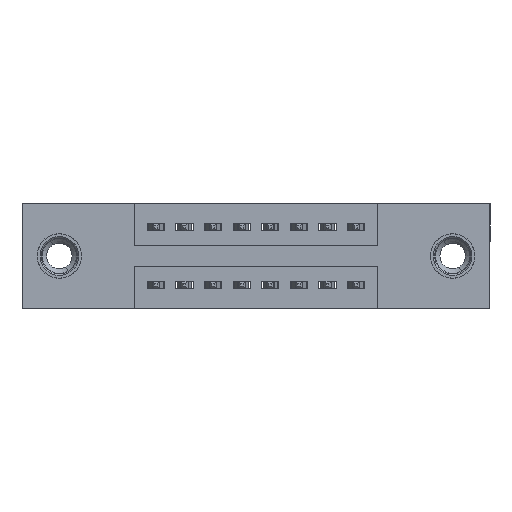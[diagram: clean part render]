
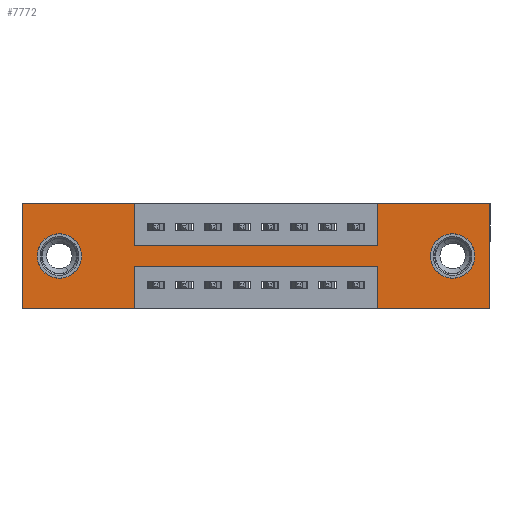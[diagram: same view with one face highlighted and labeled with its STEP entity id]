
A CAD part, front view. The second image highlights one B-rep face of the part: STEP entity #7772.
In plain terms, the highlighted planar face has unit normal (0, -1, 0).
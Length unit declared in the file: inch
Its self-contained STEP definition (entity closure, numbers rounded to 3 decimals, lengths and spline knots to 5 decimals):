
#98 = CARTESIAN_POINT ( 'NONE',  ( 1.505, 0., -0.263 ) ) ;
#171 = VERTEX_POINT ( 'NONE', #9430 ) ;
#197 = CARTESIAN_POINT ( 'NONE',  ( 0.3925, 0., -0.22 ) ) ;
#259 = CARTESIAN_POINT ( 'NONE',  ( 0.3925, 0., 0. ) ) ;
#315 = ORIENTED_EDGE ( 'NONE', *, *, #6123, .F. ) ;
#361 = ORIENTED_EDGE ( 'NONE', *, *, #10981, .F. ) ;
#428 = PLANE ( 'NONE',  #2234 ) ;
#463 = VERTEX_POINT ( 'NONE', #259 ) ;
#629 = ORIENTED_EDGE ( 'NONE', *, *, #6668, .F. ) ;
#678 = VERTEX_POINT ( 'NONE', #6455 ) ;
#683 = VERTEX_POINT ( 'NONE', #7192 ) ;
#689 = EDGE_CURVE ( 'NONE', #10946, #683, #7999, .T. ) ;
#776 = CARTESIAN_POINT ( 'NONE',  ( 1.635, 0., 0. ) ) ;
#910 = CARTESIAN_POINT ( 'NONE',  ( 0., 0., -0.37 ) ) ;
#1120 = VECTOR ( 'NONE', #7804, 39.37008 ) ;
#1314 = EDGE_LOOP ( 'NONE', ( #10425, #361, #12833, #1777, #12569, #7630, #11711, #629, #7399, #3839, #2963, #315 ) ) ;
#1713 = DIRECTION ( 'NONE',  ( 1., 0., 0. ) ) ;
#1764 = CARTESIAN_POINT ( 'NONE',  ( 1.505, 0., -0.185 ) ) ;
#1777 = ORIENTED_EDGE ( 'NONE', *, *, #10527, .F. ) ;
#1779 = DIRECTION ( 'NONE',  ( 1., 0., 0. ) ) ;
#1826 = EDGE_CURVE ( 'NONE', #463, #171, #8135, .T. ) ;
#1947 = EDGE_CURVE ( 'NONE', #9766, #4601, #3247, .T. ) ;
#1992 = DIRECTION ( 'NONE',  ( 0., 0., -1. ) ) ;
#2133 = VECTOR ( 'NONE', #1992, 39.37008 ) ;
#2201 = DIRECTION ( 'NONE',  ( 1., 0., 0. ) ) ;
#2234 = AXIS2_PLACEMENT_3D ( 'NONE', #3493, #4500, #11541 ) ;
#2265 = EDGE_CURVE ( 'NONE', #3042, #4291, #6506, .T. ) ;
#2287 = EDGE_CURVE ( 'NONE', #3822, #11981, #9197, .T. ) ;
#2395 = VECTOR ( 'NONE', #2933, 39.37008 ) ;
#2557 = CIRCLE ( 'NONE', #9091, 0.078 ) ;
#2570 = VECTOR ( 'NONE', #11744, 39.37008 ) ;
#2723 = VERTEX_POINT ( 'NONE', #5160 ) ;
#2738 = VERTEX_POINT ( 'NONE', #98 ) ;
#2766 = VERTEX_POINT ( 'NONE', #197 ) ;
#2774 = DIRECTION ( 'NONE',  ( 0., 0., -1. ) ) ;
#2791 = CARTESIAN_POINT ( 'NONE',  ( 0.13, 0., -0.263 ) ) ;
#2870 = LINE ( 'NONE', #4726, #2570 ) ;
#2933 = DIRECTION ( 'NONE',  ( -1., 0., 0. ) ) ;
#2963 = ORIENTED_EDGE ( 'NONE', *, *, #2265, .F. ) ;
#3042 = VERTEX_POINT ( 'NONE', #11651 ) ;
#3247 = CIRCLE ( 'NONE', #7638, 0.078 ) ;
#3252 = CARTESIAN_POINT ( 'NONE',  ( 0.13, 0., -0.185 ) ) ;
#3296 = FACE_OUTER_BOUND ( 'NONE', #1314, .T. ) ;
#3486 = LINE ( 'NONE', #12813, #11189 ) ;
#3493 = CARTESIAN_POINT ( 'NONE',  ( 0., 0., -0.37 ) ) ;
#3597 = FACE_BOUND ( 'NONE', #3611, .T. ) ;
#3611 = EDGE_LOOP ( 'NONE', ( #9011, #5629 ) ) ;
#3614 = CARTESIAN_POINT ( 'NONE',  ( 0.3925, 0., -0.22 ) ) ;
#3805 = VECTOR ( 'NONE', #4506, 39.37008 ) ;
#3822 = VERTEX_POINT ( 'NONE', #776 ) ;
#3839 = ORIENTED_EDGE ( 'NONE', *, *, #5457, .F. ) ;
#3974 = DIRECTION ( 'NONE',  ( -1., 0., 0. ) ) ;
#4262 = DIRECTION ( 'NONE',  ( 0., 0., 1. ) ) ;
#4291 = VERTEX_POINT ( 'NONE', #10565 ) ;
#4500 = DIRECTION ( 'NONE',  ( 0., -1., 0. ) ) ;
#4506 = DIRECTION ( 'NONE',  ( 0., 0., 1. ) ) ;
#4523 = LINE ( 'NONE', #910, #12215 ) ;
#4601 = VERTEX_POINT ( 'NONE', #7226 ) ;
#4721 = DIRECTION ( 'NONE',  ( 0., 0., 1. ) ) ;
#4726 = CARTESIAN_POINT ( 'NONE',  ( 0.3925, 0., -0.37 ) ) ;
#5076 = DIRECTION ( 'NONE',  ( 0., 0., 1. ) ) ;
#5083 = LINE ( 'NONE', #8995, #2395 ) ;
#5160 = CARTESIAN_POINT ( 'NONE',  ( 1.2425, 0., -0.22 ) ) ;
#5195 = VECTOR ( 'NONE', #2201, 39.37008 ) ;
#5441 = CARTESIAN_POINT ( 'NONE',  ( 1.505, 0., -0.185 ) ) ;
#5442 = EDGE_CURVE ( 'NONE', #2766, #7187, #2870, .T. ) ;
#5457 = EDGE_CURVE ( 'NONE', #4291, #463, #10294, .T. ) ;
#5629 = ORIENTED_EDGE ( 'NONE', *, *, #1947, .T. ) ;
#5666 = DIRECTION ( 'NONE',  ( 0., 1., 0. ) ) ;
#5895 = EDGE_CURVE ( 'NONE', #11170, #2738, #2557, .T. ) ;
#6078 = CARTESIAN_POINT ( 'NONE',  ( 0.3925, 0., 0. ) ) ;
#6123 = EDGE_CURVE ( 'NONE', #7187, #3042, #5083, .T. ) ;
#6175 = CARTESIAN_POINT ( 'NONE',  ( 0.13, 0., -0.185 ) ) ;
#6184 = CARTESIAN_POINT ( 'NONE',  ( 1.2425, 0., 0. ) ) ;
#6211 = EDGE_CURVE ( 'NONE', #678, #2723, #9187, .T. ) ;
#6443 = DIRECTION ( 'NONE',  ( 0., 0., -1. ) ) ;
#6455 = CARTESIAN_POINT ( 'NONE',  ( 1.2425, 0., -0.37 ) ) ;
#6506 = LINE ( 'NONE', #12095, #3805 ) ;
#6668 = EDGE_CURVE ( 'NONE', #171, #10946, #3486, .T. ) ;
#6863 = DIRECTION ( 'NONE',  ( 0., 0., 1. ) ) ;
#6877 = VECTOR ( 'NONE', #8703, 39.37008 ) ;
#7051 = CARTESIAN_POINT ( 'NONE',  ( 1.2425, 0., -0.37 ) ) ;
#7187 = VERTEX_POINT ( 'NONE', #8625 ) ;
#7192 = CARTESIAN_POINT ( 'NONE',  ( 1.2425, 0., 0. ) ) ;
#7226 = CARTESIAN_POINT ( 'NONE',  ( 0.13, 0., -0.107 ) ) ;
#7337 = EDGE_CURVE ( 'NONE', #2738, #11170, #8678, .T. ) ;
#7399 = ORIENTED_EDGE ( 'NONE', *, *, #1826, .F. ) ;
#7618 = EDGE_CURVE ( 'NONE', #683, #3822, #7854, .T. ) ;
#7630 = ORIENTED_EDGE ( 'NONE', *, *, #7618, .F. ) ;
#7632 = VECTOR ( 'NONE', #1713, 39.37008 ) ;
#7638 = AXIS2_PLACEMENT_3D ( 'NONE', #6175, #5666, #4721 ) ;
#7772 = ADVANCED_FACE ( 'NONE', ( #8664, #3597, #3296 ), #428, .T. ) ;
#7773 = CARTESIAN_POINT ( 'NONE',  ( 0., 0., 0. ) ) ;
#7804 = DIRECTION ( 'NONE',  ( 0., 0., -1. ) ) ;
#7854 = LINE ( 'NONE', #9276, #5195 ) ;
#7918 = CARTESIAN_POINT ( 'NONE',  ( 1.635, 0., 0. ) ) ;
#7965 = CARTESIAN_POINT ( 'NONE',  ( 1.505, 0., -0.107 ) ) ;
#7999 = LINE ( 'NONE', #6184, #10062 ) ;
#8135 = LINE ( 'NONE', #6078, #2133 ) ;
#8144 = AXIS2_PLACEMENT_3D ( 'NONE', #1764, #8840, #2774 ) ;
#8288 = EDGE_CURVE ( 'NONE', #4601, #9766, #8337, .T. ) ;
#8337 = CIRCLE ( 'NONE', #10101, 0.078 ) ;
#8593 = CARTESIAN_POINT ( 'NONE',  ( 1.635, 0., -0.37 ) ) ;
#8625 = CARTESIAN_POINT ( 'NONE',  ( 0.3925, 0., -0.37 ) ) ;
#8664 = FACE_BOUND ( 'NONE', #9076, .T. ) ;
#8678 = CIRCLE ( 'NONE', #8144, 0.078 ) ;
#8703 = DIRECTION ( 'NONE',  ( -1., 0., 0. ) ) ;
#8840 = DIRECTION ( 'NONE',  ( 0., 1., 0. ) ) ;
#8981 = ORIENTED_EDGE ( 'NONE', *, *, #7337, .T. ) ;
#8995 = CARTESIAN_POINT ( 'NONE',  ( 0., 0., -0.37 ) ) ;
#9011 = ORIENTED_EDGE ( 'NONE', *, *, #8288, .T. ) ;
#9076 = EDGE_LOOP ( 'NONE', ( #12511, #8981 ) ) ;
#9091 = AXIS2_PLACEMENT_3D ( 'NONE', #5441, #12452, #6443 ) ;
#9187 = LINE ( 'NONE', #7051, #9506 ) ;
#9197 = LINE ( 'NONE', #7918, #1120 ) ;
#9276 = CARTESIAN_POINT ( 'NONE',  ( 0., 0., 0. ) ) ;
#9430 = CARTESIAN_POINT ( 'NONE',  ( 0.3925, 0., -0.15 ) ) ;
#9506 = VECTOR ( 'NONE', #5076, 39.37008 ) ;
#9578 = LINE ( 'NONE', #3614, #6877 ) ;
#9669 = CARTESIAN_POINT ( 'NONE',  ( 1.2425, 0., -0.15 ) ) ;
#9766 = VERTEX_POINT ( 'NONE', #2791 ) ;
#10062 = VECTOR ( 'NONE', #6863, 39.37008 ) ;
#10101 = AXIS2_PLACEMENT_3D ( 'NONE', #3252, #10303, #4262 ) ;
#10294 = LINE ( 'NONE', #7773, #7632 ) ;
#10303 = DIRECTION ( 'NONE',  ( 0., 1., 0. ) ) ;
#10425 = ORIENTED_EDGE ( 'NONE', *, *, #5442, .F. ) ;
#10527 = EDGE_CURVE ( 'NONE', #11981, #678, #4523, .T. ) ;
#10565 = CARTESIAN_POINT ( 'NONE',  ( 0., 0., 0. ) ) ;
#10946 = VERTEX_POINT ( 'NONE', #9669 ) ;
#10981 = EDGE_CURVE ( 'NONE', #2723, #2766, #9578, .T. ) ;
#11170 = VERTEX_POINT ( 'NONE', #7965 ) ;
#11189 = VECTOR ( 'NONE', #1779, 39.37008 ) ;
#11541 = DIRECTION ( 'NONE',  ( 0., 0., -1. ) ) ;
#11651 = CARTESIAN_POINT ( 'NONE',  ( 0., 0., -0.37 ) ) ;
#11711 = ORIENTED_EDGE ( 'NONE', *, *, #689, .F. ) ;
#11744 = DIRECTION ( 'NONE',  ( 0., 0., -1. ) ) ;
#11981 = VERTEX_POINT ( 'NONE', #8593 ) ;
#12095 = CARTESIAN_POINT ( 'NONE',  ( 0., 0., 0. ) ) ;
#12215 = VECTOR ( 'NONE', #3974, 39.37008 ) ;
#12452 = DIRECTION ( 'NONE',  ( 0., 1., 0. ) ) ;
#12511 = ORIENTED_EDGE ( 'NONE', *, *, #5895, .T. ) ;
#12569 = ORIENTED_EDGE ( 'NONE', *, *, #2287, .F. ) ;
#12813 = CARTESIAN_POINT ( 'NONE',  ( 0.3925, 0., -0.15 ) ) ;
#12833 = ORIENTED_EDGE ( 'NONE', *, *, #6211, .F. ) ;
